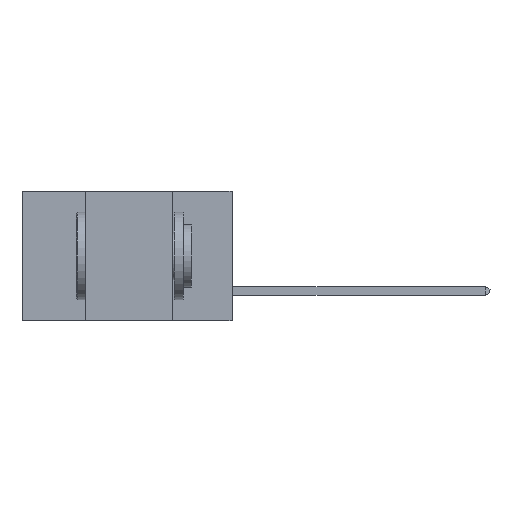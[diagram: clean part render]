
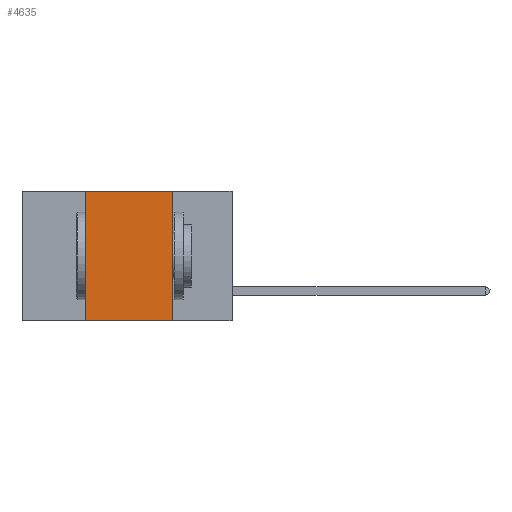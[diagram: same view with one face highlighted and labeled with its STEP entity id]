
A CAD part, left-side view. The second image highlights one B-rep face of the part: STEP entity #4635.
In plain terms, the highlighted planar face has unit normal (-1, 0, 0).
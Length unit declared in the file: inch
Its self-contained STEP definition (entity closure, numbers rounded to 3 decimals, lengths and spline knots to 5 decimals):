
#217 = LINE ( 'NONE', #2683, #2828 ) ;
#261 = DIRECTION ( 'NONE',  ( 0., 0., -1. ) ) ;
#526 = LINE ( 'NONE', #7808, #7811 ) ;
#1125 = VECTOR ( 'NONE', #10997, 39.37008 ) ;
#1475 = CARTESIAN_POINT ( 'NONE',  ( 0., 0.6, -0.37 ) ) ;
#1544 = DIRECTION ( 'NONE',  ( 0., 0., 1. ) ) ;
#1569 = ORIENTED_EDGE ( 'NONE', *, *, #6420, .F. ) ;
#1705 = EDGE_CURVE ( 'NONE', #5782, #9448, #2359, .T. ) ;
#2359 = LINE ( 'NONE', #1475, #10906 ) ;
#2621 = EDGE_LOOP ( 'NONE', ( #3733, #1569, #8743, #10683 ) ) ;
#2683 = CARTESIAN_POINT ( 'NONE',  ( 0., 0.6, 0. ) ) ;
#2828 = VECTOR ( 'NONE', #7839, 39.37008 ) ;
#3272 = CARTESIAN_POINT ( 'NONE',  ( 0., 0.17, -0.37 ) ) ;
#3733 = ORIENTED_EDGE ( 'NONE', *, *, #10260, .F. ) ;
#3915 = DIRECTION ( 'NONE',  ( 0., -1., 0. ) ) ;
#4361 = EDGE_CURVE ( 'NONE', #5782, #10706, #526, .T. ) ;
#4366 = CARTESIAN_POINT ( 'NONE',  ( 0., 0.42, -0.37 ) ) ;
#4635 = ADVANCED_FACE ( 'NONE', ( #8637 ), #10753, .F. ) ;
#5482 = CARTESIAN_POINT ( 'NONE',  ( 0., 0.17, 0. ) ) ;
#5540 = DIRECTION ( 'NONE',  ( 1., 0., 0. ) ) ;
#5782 = VERTEX_POINT ( 'NONE', #4366 ) ;
#6310 = CARTESIAN_POINT ( 'NONE',  ( 0., 0.6, 0. ) ) ;
#6420 = EDGE_CURVE ( 'NONE', #10706, #7892, #217, .T. ) ;
#7305 = LINE ( 'NONE', #5482, #1125 ) ;
#7808 = CARTESIAN_POINT ( 'NONE',  ( 0., 0.42, 0. ) ) ;
#7811 = VECTOR ( 'NONE', #1544, 39.37008 ) ;
#7839 = DIRECTION ( 'NONE',  ( 0., -1., 0. ) ) ;
#7892 = VERTEX_POINT ( 'NONE', #9251 ) ;
#7899 = CARTESIAN_POINT ( 'NONE',  ( 0., 0.42, 0. ) ) ;
#8637 = FACE_OUTER_BOUND ( 'NONE', #2621, .T. ) ;
#8743 = ORIENTED_EDGE ( 'NONE', *, *, #4361, .F. ) ;
#9251 = CARTESIAN_POINT ( 'NONE',  ( 0., 0.17, 0. ) ) ;
#9448 = VERTEX_POINT ( 'NONE', #3272 ) ;
#9518 = AXIS2_PLACEMENT_3D ( 'NONE', #6310, #5540, #261 ) ;
#10260 = EDGE_CURVE ( 'NONE', #7892, #9448, #7305, .T. ) ;
#10683 = ORIENTED_EDGE ( 'NONE', *, *, #1705, .T. ) ;
#10706 = VERTEX_POINT ( 'NONE', #7899 ) ;
#10753 = PLANE ( 'NONE',  #9518 ) ;
#10906 = VECTOR ( 'NONE', #3915, 39.37008 ) ;
#10997 = DIRECTION ( 'NONE',  ( 0., 0., -1. ) ) ;
